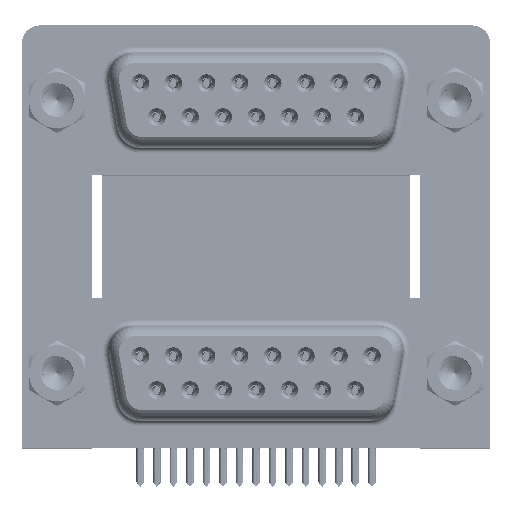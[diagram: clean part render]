
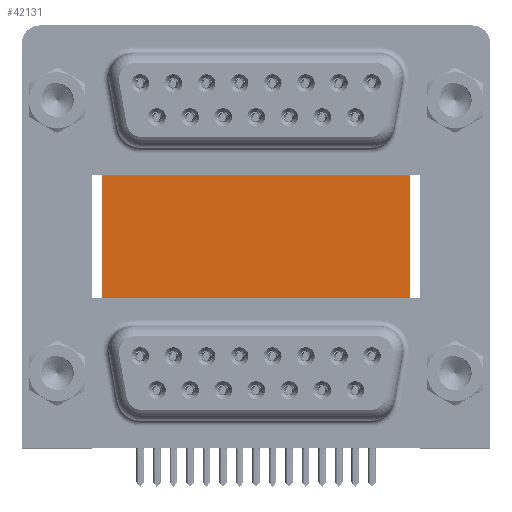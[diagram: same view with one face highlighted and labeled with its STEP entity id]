
A CAD part, top view. The second image highlights one B-rep face of the part: STEP entity #42131.
In plain terms, the highlighted planar face has unit normal (0, 0, 1).
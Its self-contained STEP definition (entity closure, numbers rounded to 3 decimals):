
#595 = CARTESIAN_POINT ( 'NONE',  ( 29.58, 16.585, -12. ) ) ;
#918 = VERTEX_POINT ( 'NONE', #31079 ) ;
#2060 = ORIENTED_EDGE ( 'NONE', *, *, #12729, .T. ) ;
#5976 = FACE_OUTER_BOUND ( 'NONE', #17102, .T. ) ;
#7256 = VERTEX_POINT ( 'NONE', #15566 ) ;
#7422 = ORIENTED_EDGE ( 'NONE', *, *, #16188, .F. ) ;
#8658 = VECTOR ( 'NONE', #42535, 1000. ) ;
#9952 = DIRECTION ( 'NONE',  ( 0., 0., -1. ) ) ;
#10885 = EDGE_CURVE ( 'NONE', #7256, #23293, #55757, .T. ) ;
#11066 = LINE ( 'NONE', #28370, #13869 ) ;
#12472 = LINE ( 'NONE', #51625, #8658 ) ;
#12729 = EDGE_CURVE ( 'NONE', #45541, #918, #11066, .T. ) ;
#13869 = VECTOR ( 'NONE', #19850, 1000. ) ;
#15566 = CARTESIAN_POINT ( 'NONE',  ( 3.79, 16.585, -12. ) ) ;
#16188 = EDGE_CURVE ( 'NONE', #23293, #918, #12472, .T. ) ;
#16412 = AXIS2_PLACEMENT_3D ( 'NONE', #49380, #9952, #53379 ) ;
#17102 = EDGE_LOOP ( 'NONE', ( #2060, #7422, #48463, #31496 ) ) ;
#19850 = DIRECTION ( 'NONE',  ( 1., 0., 0. ) ) ;
#19935 = EDGE_CURVE ( 'NONE', #7256, #45541, #24705, .T. ) ;
#22047 = VECTOR ( 'NONE', #51194, 1000. ) ;
#23293 = VERTEX_POINT ( 'NONE', #595 ) ;
#24705 = LINE ( 'NONE', #42849, #55021 ) ;
#28370 = CARTESIAN_POINT ( 'NONE',  ( 3.79, -3.735, -12. ) ) ;
#31079 = CARTESIAN_POINT ( 'NONE',  ( 29.58, -3.735, -12. ) ) ;
#31496 = ORIENTED_EDGE ( 'NONE', *, *, #19935, .T. ) ;
#37746 = DIRECTION ( 'NONE',  ( 0., -1., 0. ) ) ;
#42131 = ADVANCED_FACE ( 'NONE', ( #5976 ), #48836, .F. ) ;
#42535 = DIRECTION ( 'NONE',  ( 0., -1., 0. ) ) ;
#42673 = CARTESIAN_POINT ( 'NONE',  ( 3.79, 16.585, -12. ) ) ;
#42849 = CARTESIAN_POINT ( 'NONE',  ( 3.79, 16.585, -12. ) ) ;
#45541 = VERTEX_POINT ( 'NONE', #53606 ) ;
#48463 = ORIENTED_EDGE ( 'NONE', *, *, #10885, .F. ) ;
#48836 = PLANE ( 'NONE',  #16412 ) ;
#49380 = CARTESIAN_POINT ( 'NONE',  ( 3.79, 16.585, -12. ) ) ;
#51194 = DIRECTION ( 'NONE',  ( 1., 0., 0. ) ) ;
#51625 = CARTESIAN_POINT ( 'NONE',  ( 29.58, 16.585, -12. ) ) ;
#53379 = DIRECTION ( 'NONE',  ( -1., 0., 0. ) ) ;
#53606 = CARTESIAN_POINT ( 'NONE',  ( 3.79, -3.735, -12. ) ) ;
#55021 = VECTOR ( 'NONE', #37746, 1000. ) ;
#55757 = LINE ( 'NONE', #42673, #22047 ) ;
